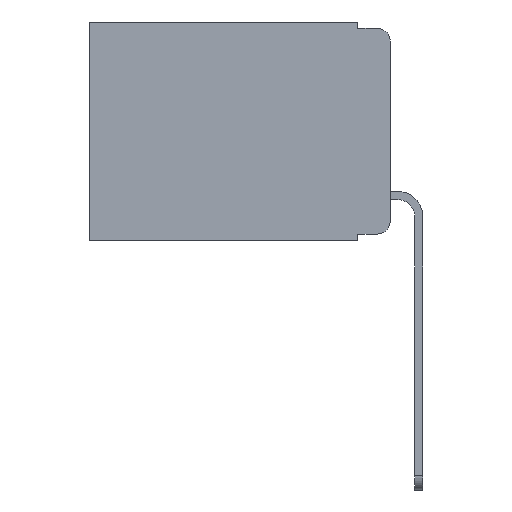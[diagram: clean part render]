
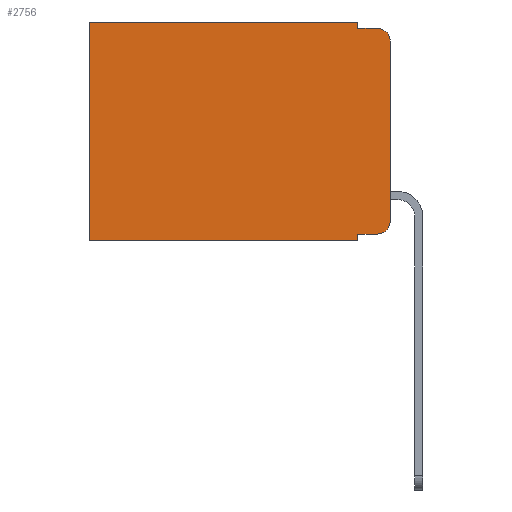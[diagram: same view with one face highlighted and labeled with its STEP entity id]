
A CAD part, left-side view. The second image highlights one B-rep face of the part: STEP entity #2756.
In plain terms, the highlighted planar face has unit normal (-1, 0, 0).
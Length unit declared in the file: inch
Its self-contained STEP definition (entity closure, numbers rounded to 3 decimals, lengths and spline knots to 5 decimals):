
#58 = DIRECTION ( 'NONE',  ( 0., -1., 0. ) ) ;
#170 = VECTOR ( 'NONE', #2754, 39.37008 ) ;
#245 = CIRCLE ( 'NONE', #8104, 0.02 ) ;
#415 = VERTEX_POINT ( 'NONE', #10368 ) ;
#900 = CARTESIAN_POINT ( 'NONE',  ( 0.298, 0.02, -0.03 ) ) ;
#903 = DIRECTION ( 'NONE',  ( -1., 0., 0. ) ) ;
#931 = DIRECTION ( 'NONE',  ( 0., 0., -1. ) ) ;
#1055 = EDGE_CURVE ( 'NONE', #8354, #5766, #7278, .T. ) ;
#1174 = LINE ( 'NONE', #4934, #10820 ) ;
#1198 = AXIS2_PLACEMENT_3D ( 'NONE', #4449, #10718, #5434 ) ;
#1259 = VERTEX_POINT ( 'NONE', #7941 ) ;
#1272 = VECTOR ( 'NONE', #58, 39.37008 ) ;
#1388 = VERTEX_POINT ( 'NONE', #11760 ) ;
#1406 = EDGE_CURVE ( 'NONE', #1388, #1259, #245, .T. ) ;
#1413 = CARTESIAN_POINT ( 'NONE',  ( 0.298, 0., 0. ) ) ;
#1793 = CARTESIAN_POINT ( 'NONE',  ( 0.298, 0., 0. ) ) ;
#1986 = VERTEX_POINT ( 'NONE', #5140 ) ;
#2000 = LINE ( 'NONE', #10550, #1272 ) ;
#2012 = PLANE ( 'NONE',  #11092 ) ;
#2069 = ORIENTED_EDGE ( 'NONE', *, *, #3925, .T. ) ;
#2116 = CARTESIAN_POINT ( 'NONE',  ( 0.298, 0.051, 0. ) ) ;
#2518 = ORIENTED_EDGE ( 'NONE', *, *, #1406, .T. ) ;
#2579 = DIRECTION ( 'NONE',  ( 0., 1., 0. ) ) ;
#2674 = DIRECTION ( 'NONE',  ( 1., 0., 0. ) ) ;
#2723 = DIRECTION ( 'NONE',  ( 0., 0., -1. ) ) ;
#2749 = DIRECTION ( 'NONE',  ( 0., 0., -1. ) ) ;
#2754 = DIRECTION ( 'NONE',  ( 0., 0., -1. ) ) ;
#2756 = ADVANCED_FACE ( 'NONE', ( #11452 ), #2012, .F. ) ;
#2834 = ORIENTED_EDGE ( 'NONE', *, *, #7776, .F. ) ;
#2890 = VECTOR ( 'NONE', #2723, 39.37008 ) ;
#3002 = VECTOR ( 'NONE', #7809, 39.37008 ) ;
#3547 = VECTOR ( 'NONE', #7204, 39.37008 ) ;
#3754 = CARTESIAN_POINT ( 'NONE',  ( 0.298, 0., 0. ) ) ;
#3773 = CARTESIAN_POINT ( 'NONE',  ( 0.298, 0.02, -0.333 ) ) ;
#3925 = EDGE_CURVE ( 'NONE', #7392, #11190, #6130, .T. ) ;
#4449 = CARTESIAN_POINT ( 'NONE',  ( 0.298, 0.02, -0.313 ) ) ;
#4549 = EDGE_CURVE ( 'NONE', #6516, #1259, #2000, .T. ) ;
#4934 = CARTESIAN_POINT ( 'NONE',  ( 0.298, 0.473, 0. ) ) ;
#5140 = CARTESIAN_POINT ( 'NONE',  ( 0.298, 0., -0.313 ) ) ;
#5162 = ORIENTED_EDGE ( 'NONE', *, *, #1055, .T. ) ;
#5389 = EDGE_CURVE ( 'NONE', #11190, #1986, #9563, .T. ) ;
#5434 = DIRECTION ( 'NONE',  ( 0., 0., -1. ) ) ;
#5442 = ORIENTED_EDGE ( 'NONE', *, *, #8076, .F. ) ;
#5580 = EDGE_CURVE ( 'NONE', #7392, #8721, #10227, .T. ) ;
#5631 = LINE ( 'NONE', #3754, #170 ) ;
#5766 = VERTEX_POINT ( 'NONE', #8610 ) ;
#5824 = DIRECTION ( 'NONE',  ( 0., 1., 0. ) ) ;
#5907 = DIRECTION ( 'NONE',  ( 0., 0., -1. ) ) ;
#6130 = LINE ( 'NONE', #9093, #3547 ) ;
#6310 = EDGE_CURVE ( 'NONE', #1388, #1986, #5631, .T. ) ;
#6468 = VECTOR ( 'NONE', #2579, 39.37008 ) ;
#6474 = CARTESIAN_POINT ( 'NONE',  ( 0.298, 0.051, -0.333 ) ) ;
#6516 = VERTEX_POINT ( 'NONE', #8598 ) ;
#7030 = EDGE_LOOP ( 'NONE', ( #11345, #2518, #11613, #2834, #5162, #8116, #5442, #10687, #2069, #11484 ) ) ;
#7204 = DIRECTION ( 'NONE',  ( 0., -1., 0. ) ) ;
#7278 = LINE ( 'NONE', #1413, #11066 ) ;
#7392 = VERTEX_POINT ( 'NONE', #6474 ) ;
#7655 = EDGE_CURVE ( 'NONE', #5766, #415, #1174, .T. ) ;
#7776 = EDGE_CURVE ( 'NONE', #8354, #6516, #11742, .T. ) ;
#7809 = DIRECTION ( 'NONE',  ( 0., 0., -1. ) ) ;
#7941 = CARTESIAN_POINT ( 'NONE',  ( 0.298, 0.02, -0.01 ) ) ;
#8076 = EDGE_CURVE ( 'NONE', #8721, #415, #8804, .T. ) ;
#8104 = AXIS2_PLACEMENT_3D ( 'NONE', #900, #903, #931 ) ;
#8116 = ORIENTED_EDGE ( 'NONE', *, *, #7655, .T. ) ;
#8354 = VERTEX_POINT ( 'NONE', #8562 ) ;
#8562 = CARTESIAN_POINT ( 'NONE',  ( 0.298, 0.051, 0. ) ) ;
#8598 = CARTESIAN_POINT ( 'NONE',  ( 0.298, 0.051, -0.01 ) ) ;
#8610 = CARTESIAN_POINT ( 'NONE',  ( 0.298, 0.473, 0. ) ) ;
#8721 = VERTEX_POINT ( 'NONE', #11460 ) ;
#8804 = LINE ( 'NONE', #10785, #6468 ) ;
#9093 = CARTESIAN_POINT ( 'NONE',  ( 0.298, 0.051, -0.333 ) ) ;
#9205 = CARTESIAN_POINT ( 'NONE',  ( 0.298, 0.051, 0. ) ) ;
#9563 = CIRCLE ( 'NONE', #1198, 0.02 ) ;
#10227 = LINE ( 'NONE', #9205, #2890 ) ;
#10368 = CARTESIAN_POINT ( 'NONE',  ( 0.298, 0.473, -0.343 ) ) ;
#10550 = CARTESIAN_POINT ( 'NONE',  ( 0.298, 0.051, -0.01 ) ) ;
#10687 = ORIENTED_EDGE ( 'NONE', *, *, #5580, .F. ) ;
#10718 = DIRECTION ( 'NONE',  ( -1., 0., 0. ) ) ;
#10785 = CARTESIAN_POINT ( 'NONE',  ( 0.298, 0., -0.343 ) ) ;
#10820 = VECTOR ( 'NONE', #5907, 39.37008 ) ;
#11066 = VECTOR ( 'NONE', #5824, 39.37008 ) ;
#11092 = AXIS2_PLACEMENT_3D ( 'NONE', #1793, #2674, #2749 ) ;
#11190 = VERTEX_POINT ( 'NONE', #3773 ) ;
#11345 = ORIENTED_EDGE ( 'NONE', *, *, #6310, .F. ) ;
#11452 = FACE_OUTER_BOUND ( 'NONE', #7030, .T. ) ;
#11460 = CARTESIAN_POINT ( 'NONE',  ( 0.298, 0.051, -0.343 ) ) ;
#11484 = ORIENTED_EDGE ( 'NONE', *, *, #5389, .T. ) ;
#11613 = ORIENTED_EDGE ( 'NONE', *, *, #4549, .F. ) ;
#11742 = LINE ( 'NONE', #2116, #3002 ) ;
#11760 = CARTESIAN_POINT ( 'NONE',  ( 0.298, 0., -0.03 ) ) ;
